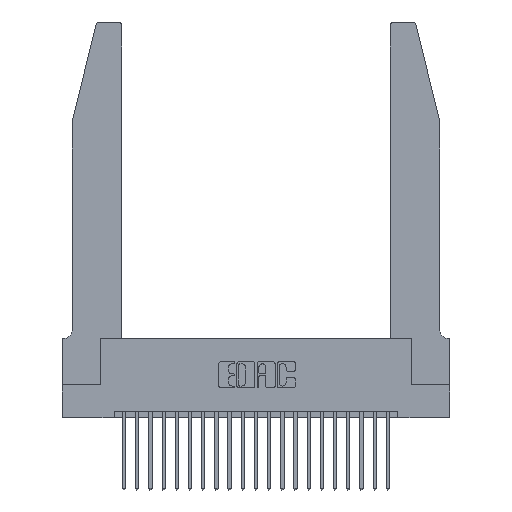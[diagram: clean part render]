
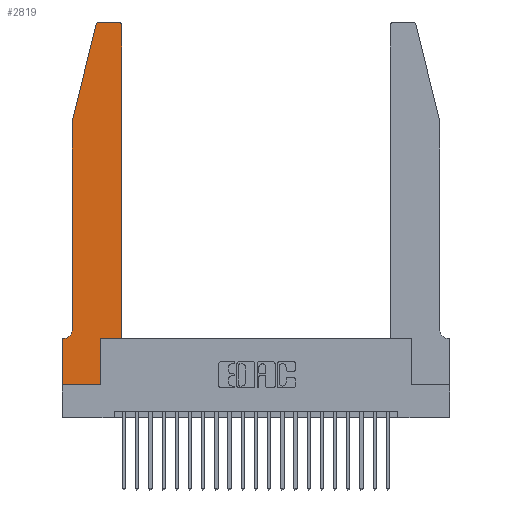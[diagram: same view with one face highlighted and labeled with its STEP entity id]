
A CAD part, top view. The second image highlights one B-rep face of the part: STEP entity #2819.
In plain terms, the highlighted planar face has unit normal (0, 0, 1).
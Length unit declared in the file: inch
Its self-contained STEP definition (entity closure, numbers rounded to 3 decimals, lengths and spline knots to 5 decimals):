
#159 = EDGE_CURVE ( 'NONE', #11859, #20676, #1111, .T. ) ;
#251 = CARTESIAN_POINT ( 'NONE',  ( 0.4205, 2.75, 0.37 ) ) ;
#344 = EDGE_CURVE ( 'NONE', #11917, #8033, #22327, .T. ) ;
#352 = AXIS2_PLACEMENT_3D ( 'NONE', #19738, #8768, #21537 ) ;
#504 = DIRECTION ( 'NONE',  ( 0., -1., 0. ) ) ;
#640 = ORIENTED_EDGE ( 'NONE', *, *, #23729, .T. ) ;
#737 = AXIS2_PLACEMENT_3D ( 'NONE', #15263, #4016, #17087 ) ;
#891 = ORIENTED_EDGE ( 'NONE', *, *, #11064, .T. ) ;
#1073 = CARTESIAN_POINT ( 'NONE',  ( 0.4505, 0.35, 0.37 ) ) ;
#1111 = LINE ( 'NONE', #3326, #15608 ) ;
#1402 = ORIENTED_EDGE ( 'NONE', *, *, #344, .T. ) ;
#1420 = EDGE_CURVE ( 'NONE', #4799, #11917, #1972, .T. ) ;
#1730 = CARTESIAN_POINT ( 'NONE',  ( 0.0755, 0.35, 0.37 ) ) ;
#1972 = LINE ( 'NONE', #1730, #6518 ) ;
#2011 = CARTESIAN_POINT ( 'NONE',  ( 0.284, 2.72, 0.37 ) ) ;
#2325 = LINE ( 'NONE', #3432, #12420 ) ;
#2740 = CARTESIAN_POINT ( 'NONE',  ( 0.4505, 2.72, 0.37 ) ) ;
#2819 = ADVANCED_FACE ( 'NONE', ( #21088 ), #17875, .T. ) ;
#2826 = EDGE_CURVE ( 'NONE', #17539, #11281, #11435, .T. ) ;
#3030 = VERTEX_POINT ( 'NONE', #17774 ) ;
#3326 = CARTESIAN_POINT ( 'NONE',  ( 0.4505, 0.35, 0.37 ) ) ;
#3356 = VECTOR ( 'NONE', #16173, 39.37008 ) ;
#3432 = CARTESIAN_POINT ( 'NONE',  ( 0., 0., 0.37 ) ) ;
#3581 = CARTESIAN_POINT ( 'NONE',  ( 0.284, 2.75, 0.37 ) ) ;
#3958 = DIRECTION ( 'NONE',  ( 1., 0., 0. ) ) ;
#4016 = DIRECTION ( 'NONE',  ( 0., 0., -1. ) ) ;
#4105 = VECTOR ( 'NONE', #9972, 39.37008 ) ;
#4799 = VERTEX_POINT ( 'NONE', #21498 ) ;
#5929 = DIRECTION ( 'NONE',  ( 0., 1., 0. ) ) ;
#6477 = EDGE_CURVE ( 'NONE', #12312, #7577, #9769, .T. ) ;
#6518 = VECTOR ( 'NONE', #9209, 39.37008 ) ;
#6644 = CARTESIAN_POINT ( 'NONE',  ( 0.2605, 2.75, 0.37 ) ) ;
#6754 = CIRCLE ( 'NONE', #352, 0.03 ) ;
#6769 = ORIENTED_EDGE ( 'NONE', *, *, #11456, .T. ) ;
#6983 = DIRECTION ( 'NONE',  ( 1., 0., 0. ) ) ;
#7577 = VERTEX_POINT ( 'NONE', #16249 ) ;
#7800 = CARTESIAN_POINT ( 'NONE',  ( 0.0755, 2., 0.37 ) ) ;
#8033 = VERTEX_POINT ( 'NONE', #19600 ) ;
#8764 = DIRECTION ( 'NONE',  ( 0., -1., 0. ) ) ;
#8768 = DIRECTION ( 'NONE',  ( 0., 0., 1. ) ) ;
#8926 = AXIS2_PLACEMENT_3D ( 'NONE', #18826, #19526, #6983 ) ;
#9096 = LINE ( 'NONE', #20975, #18285 ) ;
#9209 = DIRECTION ( 'NONE',  ( -1., 0., 0. ) ) ;
#9303 = ORIENTED_EDGE ( 'NONE', *, *, #2826, .T. ) ;
#9412 = EDGE_CURVE ( 'NONE', #7577, #11859, #21866, .T. ) ;
#9769 = LINE ( 'NONE', #19086, #4105 ) ;
#9972 = DIRECTION ( 'NONE',  ( 0., 1., 0. ) ) ;
#10522 = CARTESIAN_POINT ( 'NONE',  ( 0.25487, 2.72718, 0.37 ) ) ;
#10796 = VERTEX_POINT ( 'NONE', #11798 ) ;
#11064 = EDGE_CURVE ( 'NONE', #20676, #17539, #6754, .T. ) ;
#11281 = VERTEX_POINT ( 'NONE', #3581 ) ;
#11435 = LINE ( 'NONE', #6644, #20530 ) ;
#11456 = EDGE_CURVE ( 'NONE', #10796, #3030, #9096, .T. ) ;
#11798 = CARTESIAN_POINT ( 'NONE',  ( 0.0755, 2., 0.37 ) ) ;
#11859 = VERTEX_POINT ( 'NONE', #18538 ) ;
#11917 = VERTEX_POINT ( 'NONE', #22212 ) ;
#12312 = VERTEX_POINT ( 'NONE', #23550 ) ;
#12420 = VECTOR ( 'NONE', #16533, 39.37008 ) ;
#13319 = AXIS2_PLACEMENT_3D ( 'NONE', #2011, #15209, #3958 ) ;
#13499 = ORIENTED_EDGE ( 'NONE', *, *, #9412, .T. ) ;
#14203 = CIRCLE ( 'NONE', #737, 0.07 ) ;
#14388 = CIRCLE ( 'NONE', #13319, 0.03 ) ;
#14593 = EDGE_CURVE ( 'NONE', #3030, #4799, #14203, .T. ) ;
#15209 = DIRECTION ( 'NONE',  ( 0., 0., 1. ) ) ;
#15263 = CARTESIAN_POINT ( 'NONE',  ( 0.0055, 0.42, 0.37 ) ) ;
#15608 = VECTOR ( 'NONE', #5929, 39.37008 ) ;
#15609 = EDGE_CURVE ( 'NONE', #8033, #12312, #2325, .T. ) ;
#16173 = DIRECTION ( 'NONE',  ( 1., 0., 0. ) ) ;
#16249 = CARTESIAN_POINT ( 'NONE',  ( 0.2865, 0.35, 0.37 ) ) ;
#16533 = DIRECTION ( 'NONE',  ( 1., 0., 0. ) ) ;
#17004 = VECTOR ( 'NONE', #8764, 39.37008 ) ;
#17087 = DIRECTION ( 'NONE',  ( -1., 0., 0. ) ) ;
#17539 = VERTEX_POINT ( 'NONE', #251 ) ;
#17570 = ORIENTED_EDGE ( 'NONE', *, *, #14593, .T. ) ;
#17774 = CARTESIAN_POINT ( 'NONE',  ( 0.0755, 0.42, 0.37 ) ) ;
#17875 = PLANE ( 'NONE',  #8926 ) ;
#18285 = VECTOR ( 'NONE', #504, 39.37008 ) ;
#18381 = VECTOR ( 'NONE', #18842, 39.37008 ) ;
#18460 = CARTESIAN_POINT ( 'NONE',  ( 0., 0., 0.37 ) ) ;
#18538 = CARTESIAN_POINT ( 'NONE',  ( 0.4505, 0.35, 0.37 ) ) ;
#18826 = CARTESIAN_POINT ( 'NONE',  ( 0., 0.35, 0.37 ) ) ;
#18842 = DIRECTION ( 'NONE',  ( -0.239, -0.971, 0. ) ) ;
#19086 = CARTESIAN_POINT ( 'NONE',  ( 0.2865, 0.35, 0.37 ) ) ;
#19526 = DIRECTION ( 'NONE',  ( 0., 0., 1. ) ) ;
#19600 = CARTESIAN_POINT ( 'NONE',  ( 0., 0., 0.37 ) ) ;
#19738 = CARTESIAN_POINT ( 'NONE',  ( 0.4205, 2.72, 0.37 ) ) ;
#19867 = EDGE_CURVE ( 'NONE', #11281, #23264, #14388, .T. ) ;
#20010 = ORIENTED_EDGE ( 'NONE', *, *, #19867, .T. ) ;
#20050 = ORIENTED_EDGE ( 'NONE', *, *, #1420, .T. ) ;
#20070 = LINE ( 'NONE', #7800, #18381 ) ;
#20530 = VECTOR ( 'NONE', #21209, 39.37008 ) ;
#20676 = VERTEX_POINT ( 'NONE', #2740 ) ;
#20955 = ORIENTED_EDGE ( 'NONE', *, *, #6477, .T. ) ;
#20975 = CARTESIAN_POINT ( 'NONE',  ( 0.0755, 2., 0.37 ) ) ;
#21088 = FACE_OUTER_BOUND ( 'NONE', #22344, .T. ) ;
#21209 = DIRECTION ( 'NONE',  ( -1., 0., 0. ) ) ;
#21498 = CARTESIAN_POINT ( 'NONE',  ( 0.0055, 0.35, 0.37 ) ) ;
#21537 = DIRECTION ( 'NONE',  ( 1., 0., 0. ) ) ;
#21866 = LINE ( 'NONE', #1073, #3356 ) ;
#22042 = ORIENTED_EDGE ( 'NONE', *, *, #15609, .T. ) ;
#22119 = ORIENTED_EDGE ( 'NONE', *, *, #159, .T. ) ;
#22212 = CARTESIAN_POINT ( 'NONE',  ( 0., 0.35, 0.37 ) ) ;
#22327 = LINE ( 'NONE', #18460, #17004 ) ;
#22344 = EDGE_LOOP ( 'NONE', ( #9303, #20010, #640, #6769, #17570, #20050, #1402, #22042, #20955, #13499, #22119, #891 ) ) ;
#23264 = VERTEX_POINT ( 'NONE', #10522 ) ;
#23550 = CARTESIAN_POINT ( 'NONE',  ( 0.2865, 0., 0.37 ) ) ;
#23729 = EDGE_CURVE ( 'NONE', #23264, #10796, #20070, .T. ) ;
